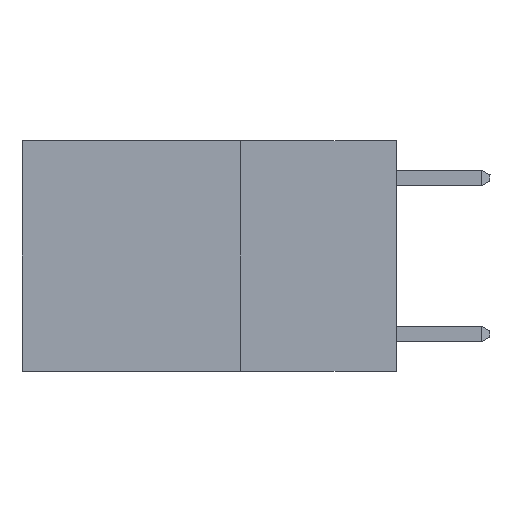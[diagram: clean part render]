
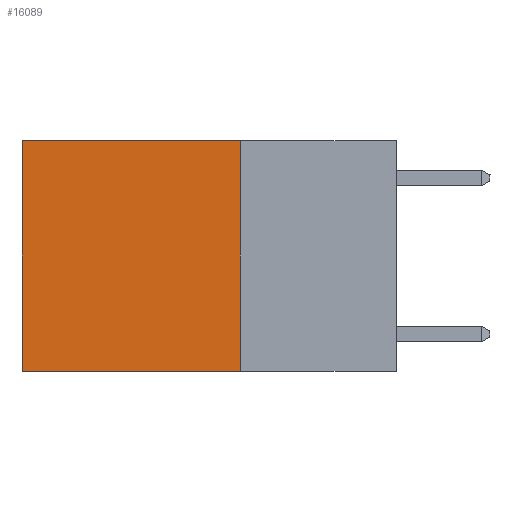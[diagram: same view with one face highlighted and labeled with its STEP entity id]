
A CAD part, left-side view. The second image highlights one B-rep face of the part: STEP entity #16089.
In plain terms, the highlighted planar face has unit normal (-1, 0, 0).
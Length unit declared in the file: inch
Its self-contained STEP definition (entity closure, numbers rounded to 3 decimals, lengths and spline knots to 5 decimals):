
#12 = VERTEX_POINT ( 'NONE', #6378 ) ;
#811 = LINE ( 'NONE', #4955, #4145 ) ;
#959 = CARTESIAN_POINT ( 'NONE',  ( 0.2625, 0.25, 0. ) ) ;
#2077 = CARTESIAN_POINT ( 'NONE',  ( 0.2625, 0.25, 0. ) ) ;
#2437 = EDGE_CURVE ( 'NONE', #12809, #11933, #2619, .T. ) ;
#2514 = CARTESIAN_POINT ( 'NONE',  ( 0.2625, 0.6, 0. ) ) ;
#2619 = LINE ( 'NONE', #10022, #6025 ) ;
#3284 = CARTESIAN_POINT ( 'NONE',  ( 0.2625, 0.25, 0. ) ) ;
#3827 = DIRECTION ( 'NONE',  ( 1., 0., 0. ) ) ;
#4145 = VECTOR ( 'NONE', #11966, 39.37008 ) ;
#4384 = VECTOR ( 'NONE', #12014, 39.37008 ) ;
#4955 = CARTESIAN_POINT ( 'NONE',  ( 0.2625, 0.25, 0. ) ) ;
#5107 = AXIS2_PLACEMENT_3D ( 'NONE', #959, #3827, #13700 ) ;
#5718 = ORIENTED_EDGE ( 'NONE', *, *, #2437, .T. ) ;
#6025 = VECTOR ( 'NONE', #11403, 39.37008 ) ;
#6378 = CARTESIAN_POINT ( 'NONE',  ( 0.2625, 0.25, -0.37 ) ) ;
#6813 = EDGE_CURVE ( 'NONE', #12, #11933, #7163, .T. ) ;
#7099 = FACE_OUTER_BOUND ( 'NONE', #13137, .T. ) ;
#7163 = LINE ( 'NONE', #10386, #10469 ) ;
#7746 = LINE ( 'NONE', #2077, #4384 ) ;
#7948 = EDGE_CURVE ( 'NONE', #17096, #12809, #7746, .T. ) ;
#8138 = EDGE_CURVE ( 'NONE', #17096, #12, #811, .T. ) ;
#8786 = ORIENTED_EDGE ( 'NONE', *, *, #8138, .F. ) ;
#9091 = DIRECTION ( 'NONE',  ( 0., 1., 0. ) ) ;
#10022 = CARTESIAN_POINT ( 'NONE',  ( 0.2625, 0.6, 0. ) ) ;
#10076 = ORIENTED_EDGE ( 'NONE', *, *, #7948, .T. ) ;
#10386 = CARTESIAN_POINT ( 'NONE',  ( 0.2625, 0.25, -0.37 ) ) ;
#10469 = VECTOR ( 'NONE', #9091, 39.37008 ) ;
#11403 = DIRECTION ( 'NONE',  ( 0., 0., -1. ) ) ;
#11933 = VERTEX_POINT ( 'NONE', #17600 ) ;
#11966 = DIRECTION ( 'NONE',  ( 0., 0., -1. ) ) ;
#12014 = DIRECTION ( 'NONE',  ( 0., 1., 0. ) ) ;
#12809 = VERTEX_POINT ( 'NONE', #2514 ) ;
#13137 = EDGE_LOOP ( 'NONE', ( #5718, #14506, #8786, #10076 ) ) ;
#13700 = DIRECTION ( 'NONE',  ( 0., 0., -1. ) ) ;
#14506 = ORIENTED_EDGE ( 'NONE', *, *, #6813, .F. ) ;
#16089 = ADVANCED_FACE ( 'NONE', ( #7099 ), #16540, .F. ) ;
#16540 = PLANE ( 'NONE',  #5107 ) ;
#17096 = VERTEX_POINT ( 'NONE', #3284 ) ;
#17600 = CARTESIAN_POINT ( 'NONE',  ( 0.2625, 0.6, -0.37 ) ) ;
